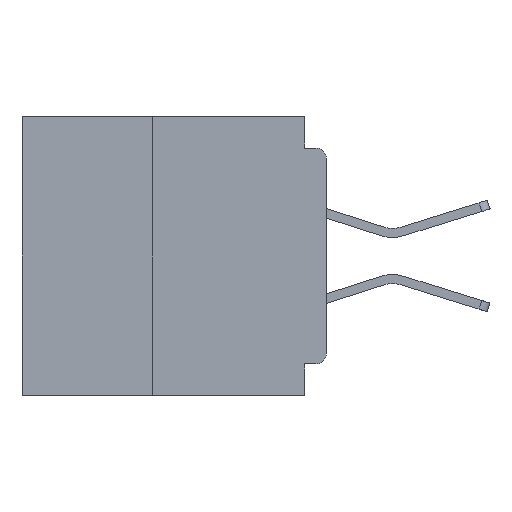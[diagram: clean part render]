
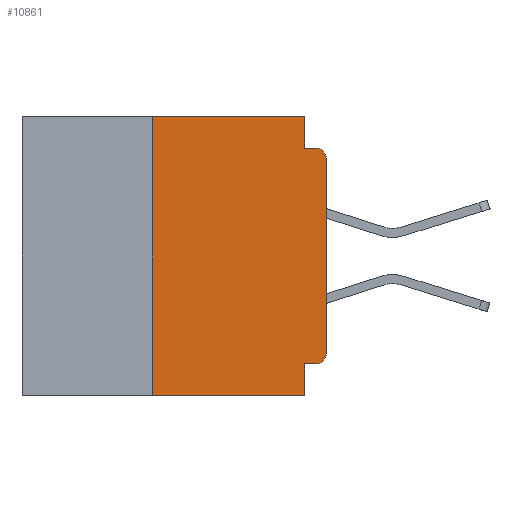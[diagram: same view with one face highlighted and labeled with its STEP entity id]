
A CAD part, left-side view. The second image highlights one B-rep face of the part: STEP entity #10861.
In plain terms, the highlighted planar face has unit normal (-1, 0, 0).
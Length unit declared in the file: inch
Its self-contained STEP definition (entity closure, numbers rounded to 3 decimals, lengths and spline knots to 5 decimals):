
#234 = LINE ( 'NONE', #2373, #32476 ) ;
#1582 = ORIENTED_EDGE ( 'NONE', *, *, #9771, .T. ) ;
#1640 = CARTESIAN_POINT ( 'NONE',  ( 0., 0.437, 0. ) ) ;
#2373 = CARTESIAN_POINT ( 'NONE',  ( 0., 0., -0.355 ) ) ;
#4562 = PLANE ( 'NONE',  #22436 ) ;
#4686 = ORIENTED_EDGE ( 'NONE', *, *, #33350, .T. ) ;
#5218 = CARTESIAN_POINT ( 'NONE',  ( 0., 0., -0.045 ) ) ;
#6207 = CARTESIAN_POINT ( 'NONE',  ( 0., 0.031, -0.4 ) ) ;
#7196 = EDGE_LOOP ( 'NONE', ( #4686, #21913, #28231, #44019, #12229, #20781, #1582, #27093, #12446, #10752 ) ) ;
#7249 = LINE ( 'NONE', #39371, #39403 ) ;
#7572 = CARTESIAN_POINT ( 'NONE',  ( 0., 0.031, -0.045 ) ) ;
#7787 = LINE ( 'NONE', #1640, #38639 ) ;
#8014 = EDGE_CURVE ( 'NONE', #25857, #43426, #51987, .T. ) ;
#8799 = LINE ( 'NONE', #18181, #18702 ) ;
#8820 = DIRECTION ( 'NONE',  ( 0., 0., -1. ) ) ;
#9481 = DIRECTION ( 'NONE',  ( 0., -1., 0. ) ) ;
#9673 = DIRECTION ( 'NONE',  ( 0., 0., -1. ) ) ;
#9771 = EDGE_CURVE ( 'NONE', #38880, #45879, #7249, .T. ) ;
#9797 = DIRECTION ( 'NONE',  ( -1., 0., 0. ) ) ;
#10752 = ORIENTED_EDGE ( 'NONE', *, *, #49418, .T. ) ;
#10861 = ADVANCED_FACE ( 'NONE', ( #41469 ), #4562, .F. ) ;
#10959 = VERTEX_POINT ( 'NONE', #26114 ) ;
#12229 = ORIENTED_EDGE ( 'NONE', *, *, #46104, .F. ) ;
#12429 = CARTESIAN_POINT ( 'NONE',  ( 0., 0.031, 0. ) ) ;
#12443 = LINE ( 'NONE', #19406, #33448 ) ;
#12446 = ORIENTED_EDGE ( 'NONE', *, *, #31581, .F. ) ;
#12560 = CARTESIAN_POINT ( 'NONE',  ( 0., 0., -0.34 ) ) ;
#14649 = LINE ( 'NONE', #52332, #45411 ) ;
#14712 = EDGE_CURVE ( 'NONE', #31965, #43426, #18885, .T. ) ;
#14722 = DIRECTION ( 'NONE',  ( 0., 0., -1. ) ) ;
#15143 = DIRECTION ( 'NONE',  ( 0., 0., 1. ) ) ;
#17074 = VERTEX_POINT ( 'NONE', #12560 ) ;
#17151 = CARTESIAN_POINT ( 'NONE',  ( 0., 0.437, 0. ) ) ;
#18181 = CARTESIAN_POINT ( 'NONE',  ( 0., 0.031, 0. ) ) ;
#18702 = VECTOR ( 'NONE', #9673, 39.37008 ) ;
#18885 = CIRCLE ( 'NONE', #26439, 0.015 ) ;
#19208 = DIRECTION ( 'NONE',  ( 0., 1., 0. ) ) ;
#19406 = CARTESIAN_POINT ( 'NONE',  ( 0., 0.25, -0.4 ) ) ;
#20781 = ORIENTED_EDGE ( 'NONE', *, *, #25664, .F. ) ;
#21913 = ORIENTED_EDGE ( 'NONE', *, *, #14712, .T. ) ;
#21972 = DIRECTION ( 'NONE',  ( -1., 0., 0. ) ) ;
#22436 = AXIS2_PLACEMENT_3D ( 'NONE', #17151, #33972, #8820 ) ;
#24714 = VECTOR ( 'NONE', #14722, 39.37008 ) ;
#25664 = EDGE_CURVE ( 'NONE', #38880, #10959, #12443, .T. ) ;
#25857 = VERTEX_POINT ( 'NONE', #7572 ) ;
#26114 = CARTESIAN_POINT ( 'NONE',  ( 0., 0.25, 0. ) ) ;
#26439 = AXIS2_PLACEMENT_3D ( 'NONE', #34932, #9797, #39145 ) ;
#26955 = DIRECTION ( 'NONE',  ( 0., -1., 0. ) ) ;
#26967 = CARTESIAN_POINT ( 'NONE',  ( 0., 0.031, -0.355 ) ) ;
#27093 = ORIENTED_EDGE ( 'NONE', *, *, #53138, .F. ) ;
#27387 = DIRECTION ( 'NONE',  ( 0., 0., 1. ) ) ;
#28231 = ORIENTED_EDGE ( 'NONE', *, *, #8014, .F. ) ;
#29499 = CARTESIAN_POINT ( 'NONE',  ( 0., 0.031, -0.4 ) ) ;
#29596 = VERTEX_POINT ( 'NONE', #12429 ) ;
#30916 = CARTESIAN_POINT ( 'NONE',  ( 0., 0.25, -0.4 ) ) ;
#31581 = EDGE_CURVE ( 'NONE', #44893, #47281, #234, .T. ) ;
#31583 = CARTESIAN_POINT ( 'NONE',  ( 0., 0.015, -0.355 ) ) ;
#31965 = VERTEX_POINT ( 'NONE', #46739 ) ;
#32476 = VECTOR ( 'NONE', #19208, 39.37008 ) ;
#32744 = AXIS2_PLACEMENT_3D ( 'NONE', #46954, #21972, #51141 ) ;
#33350 = EDGE_CURVE ( 'NONE', #17074, #31965, #14649, .T. ) ;
#33448 = VECTOR ( 'NONE', #15143, 39.37008 ) ;
#33972 = DIRECTION ( 'NONE',  ( 1., 0., 0. ) ) ;
#34932 = CARTESIAN_POINT ( 'NONE',  ( 0., 0.015, -0.06 ) ) ;
#38639 = VECTOR ( 'NONE', #39491, 39.37008 ) ;
#38880 = VERTEX_POINT ( 'NONE', #30916 ) ;
#39145 = DIRECTION ( 'NONE',  ( 0., 0., -1. ) ) ;
#39371 = CARTESIAN_POINT ( 'NONE',  ( 0., 0.437, -0.4 ) ) ;
#39403 = VECTOR ( 'NONE', #26955, 39.37008 ) ;
#39491 = DIRECTION ( 'NONE',  ( 0., -1., 0. ) ) ;
#40940 = VECTOR ( 'NONE', #9481, 39.37008 ) ;
#41469 = FACE_OUTER_BOUND ( 'NONE', #7196, .T. ) ;
#43144 = EDGE_CURVE ( 'NONE', #29596, #25857, #8799, .T. ) ;
#43426 = VERTEX_POINT ( 'NONE', #49191 ) ;
#44019 = ORIENTED_EDGE ( 'NONE', *, *, #43144, .F. ) ;
#44893 = VERTEX_POINT ( 'NONE', #31583 ) ;
#45411 = VECTOR ( 'NONE', #27387, 39.37008 ) ;
#45879 = VERTEX_POINT ( 'NONE', #29499 ) ;
#46104 = EDGE_CURVE ( 'NONE', #10959, #29596, #7787, .T. ) ;
#46739 = CARTESIAN_POINT ( 'NONE',  ( 0., 0., -0.06 ) ) ;
#46916 = LINE ( 'NONE', #6207, #24714 ) ;
#46954 = CARTESIAN_POINT ( 'NONE',  ( 0., 0.015, -0.34 ) ) ;
#47281 = VERTEX_POINT ( 'NONE', #26967 ) ;
#49191 = CARTESIAN_POINT ( 'NONE',  ( 0., 0.015, -0.045 ) ) ;
#49418 = EDGE_CURVE ( 'NONE', #44893, #17074, #51589, .T. ) ;
#51141 = DIRECTION ( 'NONE',  ( 0., 0., -1. ) ) ;
#51589 = CIRCLE ( 'NONE', #32744, 0.015 ) ;
#51987 = LINE ( 'NONE', #5218, #40940 ) ;
#52332 = CARTESIAN_POINT ( 'NONE',  ( 0., 0., 0. ) ) ;
#53138 = EDGE_CURVE ( 'NONE', #47281, #45879, #46916, .T. ) ;
